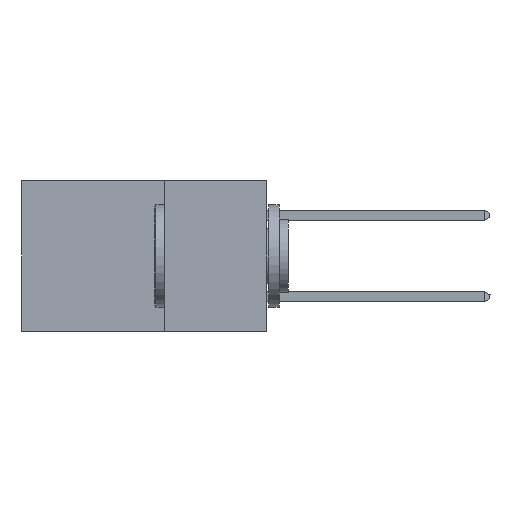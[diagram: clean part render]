
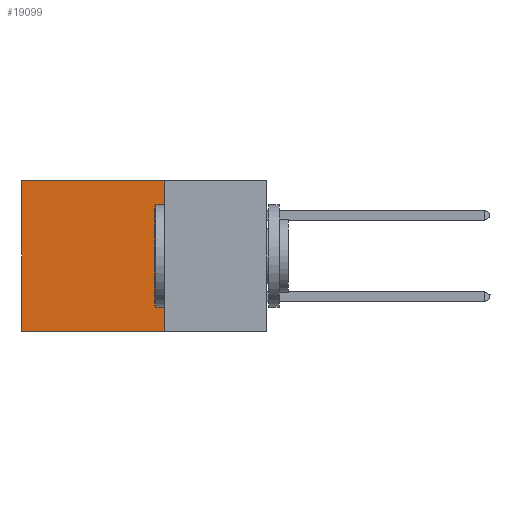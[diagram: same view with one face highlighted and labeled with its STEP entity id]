
A CAD part, left-side view. The second image highlights one B-rep face of the part: STEP entity #19099.
In plain terms, the highlighted planar face has unit normal (-1, 0, 0).
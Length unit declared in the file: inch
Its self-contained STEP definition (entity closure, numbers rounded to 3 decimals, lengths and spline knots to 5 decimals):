
#393 = VECTOR ( 'NONE', #18994, 39.37008 ) ;
#630 = VECTOR ( 'NONE', #12234, 39.37008 ) ;
#703 = LINE ( 'NONE', #7514, #14478 ) ;
#1077 = EDGE_LOOP ( 'NONE', ( #19914, #9804, #11156, #6108 ) ) ;
#1435 = CARTESIAN_POINT ( 'NONE',  ( 0.2875, 0.25, -0.37 ) ) ;
#1443 = EDGE_CURVE ( 'NONE', #6777, #2272, #703, .T. ) ;
#2272 = VERTEX_POINT ( 'NONE', #14322 ) ;
#2908 = FACE_OUTER_BOUND ( 'NONE', #1077, .T. ) ;
#4428 = DIRECTION ( 'NONE',  ( 0., 0., -1. ) ) ;
#4642 = DIRECTION ( 'NONE',  ( 1., 0., 0. ) ) ;
#4719 = DIRECTION ( 'NONE',  ( 0., 0., -1. ) ) ;
#5859 = VERTEX_POINT ( 'NONE', #14964 ) ;
#5929 = EDGE_CURVE ( 'NONE', #5859, #6504, #13723, .T. ) ;
#6108 = ORIENTED_EDGE ( 'NONE', *, *, #6852, .T. ) ;
#6504 = VERTEX_POINT ( 'NONE', #16662 ) ;
#6777 = VERTEX_POINT ( 'NONE', #15931 ) ;
#6852 = EDGE_CURVE ( 'NONE', #6777, #5859, #19435, .T. ) ;
#7222 = EDGE_CURVE ( 'NONE', #2272, #6504, #15112, .T. ) ;
#7514 = CARTESIAN_POINT ( 'NONE',  ( 0.2875, 0.25, 0. ) ) ;
#9804 = ORIENTED_EDGE ( 'NONE', *, *, #7222, .F. ) ;
#10883 = DIRECTION ( 'NONE',  ( 0., 0., -1. ) ) ;
#11156 = ORIENTED_EDGE ( 'NONE', *, *, #1443, .F. ) ;
#12234 = DIRECTION ( 'NONE',  ( 0., 1., 0. ) ) ;
#13723 = LINE ( 'NONE', #16959, #19951 ) ;
#14322 = CARTESIAN_POINT ( 'NONE',  ( 0.2875, 0.25, -0.37 ) ) ;
#14478 = VECTOR ( 'NONE', #4428, 39.37008 ) ;
#14964 = CARTESIAN_POINT ( 'NONE',  ( 0.2875, 0.6, 0. ) ) ;
#15080 = AXIS2_PLACEMENT_3D ( 'NONE', #15196, #4642, #4719 ) ;
#15112 = LINE ( 'NONE', #1435, #630 ) ;
#15196 = CARTESIAN_POINT ( 'NONE',  ( 0.2875, 0.25, 0. ) ) ;
#15264 = PLANE ( 'NONE',  #15080 ) ;
#15931 = CARTESIAN_POINT ( 'NONE',  ( 0.2875, 0.25, 0. ) ) ;
#16662 = CARTESIAN_POINT ( 'NONE',  ( 0.2875, 0.6, -0.37 ) ) ;
#16959 = CARTESIAN_POINT ( 'NONE',  ( 0.2875, 0.6, 0. ) ) ;
#17299 = CARTESIAN_POINT ( 'NONE',  ( 0.2875, 0.25, 0. ) ) ;
#18994 = DIRECTION ( 'NONE',  ( 0., 1., 0. ) ) ;
#19099 = ADVANCED_FACE ( 'NONE', ( #2908 ), #15264, .F. ) ;
#19435 = LINE ( 'NONE', #17299, #393 ) ;
#19914 = ORIENTED_EDGE ( 'NONE', *, *, #5929, .T. ) ;
#19951 = VECTOR ( 'NONE', #10883, 39.37008 ) ;
